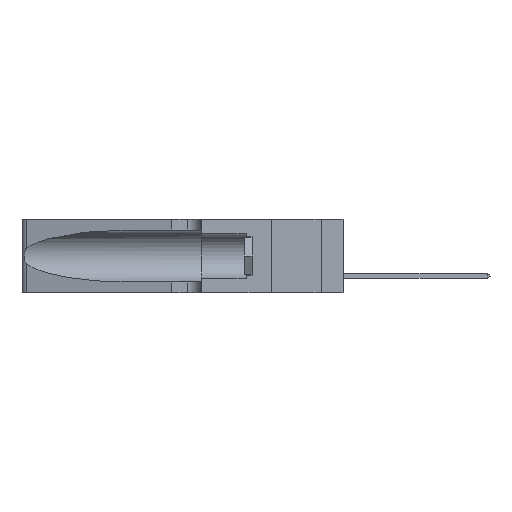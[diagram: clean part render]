
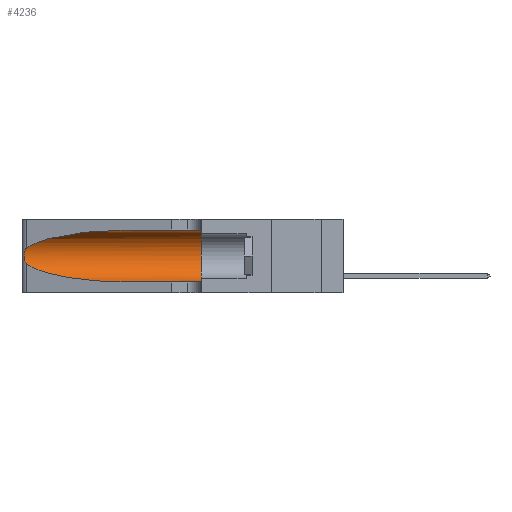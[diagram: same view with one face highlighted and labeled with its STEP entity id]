
A CAD part, left-side view. The second image highlights one B-rep face of the part: STEP entity #4236.
In plain terms, the highlighted cylindrical face has radius 3.308 mm (diameter 6.617 mm), a partial arc.
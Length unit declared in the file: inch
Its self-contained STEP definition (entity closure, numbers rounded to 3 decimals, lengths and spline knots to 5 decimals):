
#511 =( BOUNDED_CURVE ( )  B_SPLINE_CURVE ( 3, ( #29378, #854, #21463, #5812 ),
 .UNSPECIFIED., .F., .F. ) 
 B_SPLINE_CURVE_WITH_KNOTS ( ( 4, 4 ),
 ( 1.5708, 2.84003 ),
 .UNSPECIFIED. ) 
 CURVE ( )  GEOMETRIC_REPRESENTATION_ITEM ( )  RATIONAL_B_SPLINE_CURVE ( ( 1., 0.87, 0.87, 1. ) ) 
 REPRESENTATION_ITEM ( '' )  );
#854 = CARTESIAN_POINT ( 'NONE',  ( 0.18966, 0.96281, 0.31525 ) ) ;
#1236 = AXIS2_PLACEMENT_3D ( 'NONE', #4089, #22154, #32803 ) ;
#1686 = ORIENTED_EDGE ( 'NONE', *, *, #33830, .F. ) ;
#1894 = DIRECTION ( 'NONE',  ( 0., -1., 0. ) ) ;
#2710 = CARTESIAN_POINT ( 'NONE',  ( 0.25487, 1.22718, 0.14631 ) ) ;
#2931 = CARTESIAN_POINT ( 'NONE',  ( 0.18966, 0.96281, 0.05475 ) ) ;
#4089 = CARTESIAN_POINT ( 'NONE',  ( 0.1305, 1.61858, 0.185 ) ) ;
#4096 = CARTESIAN_POINT ( 'NONE',  ( 0.25487, 1.22718, 0.22369 ) ) ;
#4236 = ADVANCED_FACE ( 'NONE', ( #18857 ), #11047, .F. ) ;
#4539 = CARTESIAN_POINT ( 'NONE',  ( 0.25487, 1.22718, 0.14631 ) ) ;
#5559 = ORIENTED_EDGE ( 'NONE', *, *, #10135, .F. ) ;
#5708 = VERTEX_POINT ( 'NONE', #8610 ) ;
#5812 = CARTESIAN_POINT ( 'NONE',  ( 0.25487, 1.22718, 0.22369 ) ) ;
#6275 = CARTESIAN_POINT ( 'NONE',  ( 0.25787, 1.23484, 0.2124 ) ) ;
#6604 = ORIENTED_EDGE ( 'NONE', *, *, #22382, .T. ) ;
#6831 = CARTESIAN_POINT ( 'NONE',  ( 0.1305, 0.72297, 0.05475 ) ) ;
#6943 = CARTESIAN_POINT ( 'NONE',  ( 0.1305, 1.61858, 0.05475 ) ) ;
#7201 = CARTESIAN_POINT ( 'NONE',  ( 0.25639, 1.23186, 0.15144 ) ) ;
#7246 = EDGE_LOOP ( 'NONE', ( #20597, #11263, #30163, #6604, #1686, #5559 ) ) ;
#8369 = CARTESIAN_POINT ( 'NONE',  ( 0.1305, 0.35, 0.31525 ) ) ;
#8411 = CARTESIAN_POINT ( 'NONE',  ( 0.2373, 1.15595, 0.08982 ) ) ;
#8610 = CARTESIAN_POINT ( 'NONE',  ( 0.1305, 0.35, 0.05475 ) ) ;
#8797 = VERTEX_POINT ( 'NONE', #27639 ) ;
#8870 = CARTESIAN_POINT ( 'NONE',  ( 0.26017, 1.23833, 0.17102 ) ) ;
#10135 = EDGE_CURVE ( 'NONE', #14367, #16635, #15468, .T. ) ;
#11047 = CYLINDRICAL_SURFACE ( 'NONE', #1236, 0.13025 ) ;
#11263 = ORIENTED_EDGE ( 'NONE', *, *, #19020, .T. ) ;
#11473 = CARTESIAN_POINT ( 'NONE',  ( 0.25856, 1.23593, 0.16098 ) ) ;
#12049 = CARTESIAN_POINT ( 'NONE',  ( 0.25555, 1.22993, 0.14849 ) ) ;
#12677 = VECTOR ( 'NONE', #1894, 39.37008 ) ;
#13717 =( BOUNDED_CURVE ( )  B_SPLINE_CURVE ( 3, ( #18603, #8411, #2931, #23926 ),
 .UNSPECIFIED., .F., .T. ) 
 B_SPLINE_CURVE_WITH_KNOTS ( ( 4, 4 ),
 ( 3.44316, 4.71239 ),
 .UNSPECIFIED. ) 
 CURVE ( )  GEOMETRIC_REPRESENTATION_ITEM ( )  RATIONAL_B_SPLINE_CURVE ( ( 1., 0.87, 0.87, 1. ) ) 
 REPRESENTATION_ITEM ( '' )  );
#14239 = EDGE_CURVE ( 'NONE', #14367, #8797, #511, .T. ) ;
#14367 = VERTEX_POINT ( 'NONE', #21499 ) ;
#14724 = CARTESIAN_POINT ( 'NONE',  ( 0.1305, 0.35, 0.185 ) ) ;
#15468 = LINE ( 'NONE', #19825, #29818 ) ;
#16635 = VERTEX_POINT ( 'NONE', #8369 ) ;
#16664 = CARTESIAN_POINT ( 'NONE',  ( 0.26018, 1.23835, 0.19895 ) ) ;
#17498 = DIRECTION ( 'NONE',  ( 0., 0., 1. ) ) ;
#18603 = CARTESIAN_POINT ( 'NONE',  ( 0.25487, 1.22718, 0.14631 ) ) ;
#18857 = FACE_OUTER_BOUND ( 'NONE', #7246, .T. ) ;
#19020 = EDGE_CURVE ( 'NONE', #8797, #23116, #25983, .T. ) ;
#19825 = CARTESIAN_POINT ( 'NONE',  ( 0.1305, 1.61858, 0.31525 ) ) ;
#20137 = VERTEX_POINT ( 'NONE', #6831 ) ;
#20597 = ORIENTED_EDGE ( 'NONE', *, *, #14239, .T. ) ;
#21463 = CARTESIAN_POINT ( 'NONE',  ( 0.2373, 1.15595, 0.28018 ) ) ;
#21499 = CARTESIAN_POINT ( 'NONE',  ( 0.1305, 0.72297, 0.31525 ) ) ;
#21924 = CARTESIAN_POINT ( 'NONE',  ( 0.25854, 1.2359, 0.20912 ) ) ;
#22154 = DIRECTION ( 'NONE',  ( 0., -1., 0. ) ) ;
#22327 = DIRECTION ( 'NONE',  ( 0., -1., 0. ) ) ;
#22382 = EDGE_CURVE ( 'NONE', #20137, #5708, #31936, .T. ) ;
#22960 = AXIS2_PLACEMENT_3D ( 'NONE', #14724, #22985, #17498 ) ;
#22969 = CARTESIAN_POINT ( 'NONE',  ( 0.25789, 1.23486, 0.15765 ) ) ;
#22985 = DIRECTION ( 'NONE',  ( 0., 1., 0. ) ) ;
#23116 = VERTEX_POINT ( 'NONE', #2710 ) ;
#23926 = CARTESIAN_POINT ( 'NONE',  ( 0.1305, 0.72297, 0.05475 ) ) ;
#24310 = EDGE_CURVE ( 'NONE', #23116, #20137, #13717, .T. ) ;
#24625 = CARTESIAN_POINT ( 'NONE',  ( 0.26075, 1.23896, 0.19203 ) ) ;
#25983 = B_SPLINE_CURVE_WITH_KNOTS ( 'NONE', 3,
 ( #4096, #27117, #29733, #6275, #21924, #16664, #24625, #29845, #8870, #11473, #22969, #7201, #12049, #4539 ),
 .UNSPECIFIED., .F., .F.,
 ( 4, 2, 2, 2, 2, 2, 4 ),
 ( 0., 0.00027, 0.00053, 0.00107, 0.0016, 0.00187, 0.00214 ),
 .UNSPECIFIED. ) ;
#27117 = CARTESIAN_POINT ( 'NONE',  ( 0.25555, 1.22994, 0.2215 ) ) ;
#27639 = CARTESIAN_POINT ( 'NONE',  ( 0.25487, 1.22718, 0.22369 ) ) ;
#29378 = CARTESIAN_POINT ( 'NONE',  ( 0.1305, 0.72297, 0.31525 ) ) ;
#29733 = CARTESIAN_POINT ( 'NONE',  ( 0.25639, 1.23184, 0.21858 ) ) ;
#29818 = VECTOR ( 'NONE', #22327, 39.37008 ) ;
#29845 = CARTESIAN_POINT ( 'NONE',  ( 0.26075, 1.23896, 0.178 ) ) ;
#30163 = ORIENTED_EDGE ( 'NONE', *, *, #24310, .T. ) ;
#31936 = LINE ( 'NONE', #6943, #12677 ) ;
#32803 = DIRECTION ( 'NONE',  ( 0., 0., -1. ) ) ;
#33240 = CIRCLE ( 'NONE', #22960, 0.13025 ) ;
#33830 = EDGE_CURVE ( 'NONE', #16635, #5708, #33240, .T. ) ;
